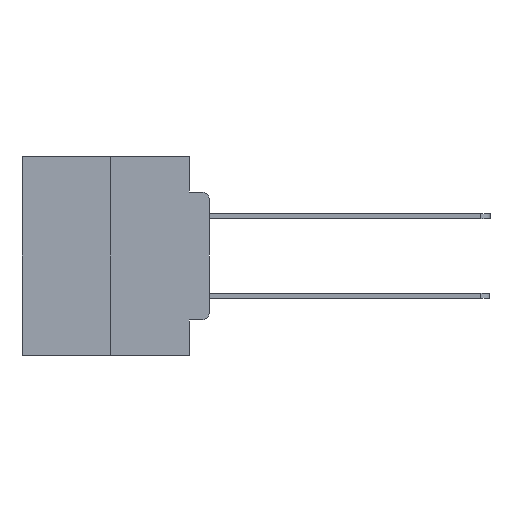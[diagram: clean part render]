
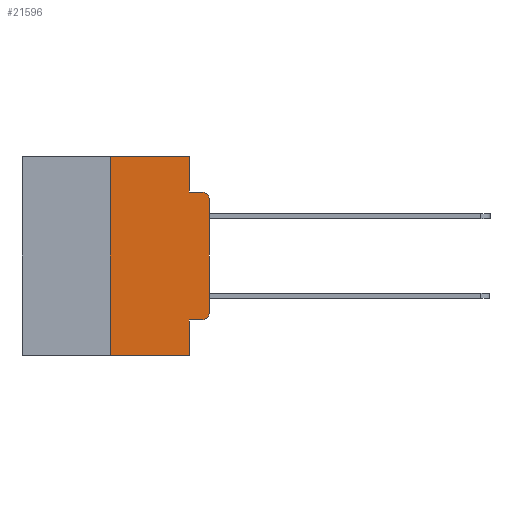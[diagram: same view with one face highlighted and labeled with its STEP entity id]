
A CAD part, left-side view. The second image highlights one B-rep face of the part: STEP entity #21596.
In plain terms, the highlighted planar face has unit normal (-1, 0, 0).
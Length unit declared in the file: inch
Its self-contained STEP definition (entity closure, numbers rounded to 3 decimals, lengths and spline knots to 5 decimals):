
#560 = EDGE_CURVE ( 'NONE', #5393, #11531, #21875, .T. ) ;
#798 = CARTESIAN_POINT ( 'NONE',  ( 0., 0., -0.1085 ) ) ;
#1005 = LINE ( 'NONE', #23950, #6911 ) ;
#1143 = LINE ( 'NONE', #4896, #27524 ) ;
#1494 = ORIENTED_EDGE ( 'NONE', *, *, #15225, .F. ) ;
#2131 = EDGE_CURVE ( 'NONE', #12512, #5947, #9195, .T. ) ;
#2373 = CARTESIAN_POINT ( 'NONE',  ( 0., 0.051, 0. ) ) ;
#2873 = AXIS2_PLACEMENT_3D ( 'NONE', #20112, #7350, #22235 ) ;
#3146 = DIRECTION ( 'NONE',  ( 0., 0., -1. ) ) ;
#3286 = VERTEX_POINT ( 'NONE', #798 ) ;
#3733 = CARTESIAN_POINT ( 'NONE',  ( 0., 0.02, -0.1085 ) ) ;
#3812 = PLANE ( 'NONE',  #27395 ) ;
#4896 = CARTESIAN_POINT ( 'NONE',  ( 0., 0.051, -0.0885 ) ) ;
#4915 = CARTESIAN_POINT ( 'NONE',  ( 0., 0.051, -0.0885 ) ) ;
#4921 = CARTESIAN_POINT ( 'NONE',  ( 0., 0.473, 0. ) ) ;
#4930 = CARTESIAN_POINT ( 'NONE',  ( 0., 0.051, 0. ) ) ;
#5388 = DIRECTION ( 'NONE',  ( 0., 0., 1. ) ) ;
#5393 = VERTEX_POINT ( 'NONE', #4930 ) ;
#5438 = DIRECTION ( 'NONE',  ( 0., 0., 1. ) ) ;
#5648 = DIRECTION ( 'NONE',  ( 0., -1., 0. ) ) ;
#5931 = DIRECTION ( 'NONE',  ( 0., 0., -1. ) ) ;
#5947 = VERTEX_POINT ( 'NONE', #11016 ) ;
#6305 = ORIENTED_EDGE ( 'NONE', *, *, #6551, .F. ) ;
#6402 = CARTESIAN_POINT ( 'NONE',  ( 0., 0.051, -0.4115 ) ) ;
#6551 = EDGE_CURVE ( 'NONE', #12512, #6640, #1005, .T. ) ;
#6640 = VERTEX_POINT ( 'NONE', #11622 ) ;
#6777 = EDGE_CURVE ( 'NONE', #8272, #3286, #12332, .T. ) ;
#6790 = FACE_OUTER_BOUND ( 'NONE', #13102, .T. ) ;
#6911 = VECTOR ( 'NONE', #17625, 39.37008 ) ;
#7350 = DIRECTION ( 'NONE',  ( -1., 0., 0. ) ) ;
#8020 = EDGE_CURVE ( 'NONE', #3286, #26626, #10301, .T. ) ;
#8272 = VERTEX_POINT ( 'NONE', #25757 ) ;
#8650 = DIRECTION ( 'NONE',  ( 0., -1., 0. ) ) ;
#9195 = LINE ( 'NONE', #10422, #19794 ) ;
#9824 = CARTESIAN_POINT ( 'NONE',  ( 0., 0., 0. ) ) ;
#9981 = VERTEX_POINT ( 'NONE', #23063 ) ;
#10078 = ORIENTED_EDGE ( 'NONE', *, *, #25552, .T. ) ;
#10301 = CIRCLE ( 'NONE', #15182, 0.02 ) ;
#10422 = CARTESIAN_POINT ( 'NONE',  ( 0., 0.051, -0.4115 ) ) ;
#10430 = ORIENTED_EDGE ( 'NONE', *, *, #27284, .T. ) ;
#11016 = CARTESIAN_POINT ( 'NONE',  ( 0., 0.02, -0.4115 ) ) ;
#11531 = VERTEX_POINT ( 'NONE', #4915 ) ;
#11622 = CARTESIAN_POINT ( 'NONE',  ( 0., 0.051, -0.5 ) ) ;
#12332 = LINE ( 'NONE', #9824, #22879 ) ;
#12512 = VERTEX_POINT ( 'NONE', #6402 ) ;
#12533 = DIRECTION ( 'NONE',  ( 0., 0., -1. ) ) ;
#13102 = EDGE_LOOP ( 'NONE', ( #17029, #13555, #16099, #14745, #20317, #1494, #10430, #6305, #27192, #10078 ) ) ;
#13258 = CARTESIAN_POINT ( 'NONE',  ( 0., 0.25, -0.5 ) ) ;
#13261 = VERTEX_POINT ( 'NONE', #13258 ) ;
#13336 = EDGE_CURVE ( 'NONE', #9981, #5393, #16441, .T. ) ;
#13555 = ORIENTED_EDGE ( 'NONE', *, *, #8020, .T. ) ;
#13775 = EDGE_CURVE ( 'NONE', #11531, #26626, #1143, .T. ) ;
#13979 = CARTESIAN_POINT ( 'NONE',  ( 0., 0.25, 0. ) ) ;
#14745 = ORIENTED_EDGE ( 'NONE', *, *, #560, .F. ) ;
#15182 = AXIS2_PLACEMENT_3D ( 'NONE', #3733, #18704, #5931 ) ;
#15225 = EDGE_CURVE ( 'NONE', #13261, #9981, #24836, .T. ) ;
#16099 = ORIENTED_EDGE ( 'NONE', *, *, #13775, .F. ) ;
#16441 = LINE ( 'NONE', #4921, #21406 ) ;
#17029 = ORIENTED_EDGE ( 'NONE', *, *, #6777, .T. ) ;
#17625 = DIRECTION ( 'NONE',  ( 0., 0., -1. ) ) ;
#17728 = DIRECTION ( 'NONE',  ( 0., -1., 0. ) ) ;
#18704 = DIRECTION ( 'NONE',  ( -1., 0., 0. ) ) ;
#19106 = CIRCLE ( 'NONE', #2873, 0.02 ) ;
#19290 = VECTOR ( 'NONE', #5388, 39.37008 ) ;
#19794 = VECTOR ( 'NONE', #5648, 39.37008 ) ;
#19862 = DIRECTION ( 'NONE',  ( 0., -1., 0. ) ) ;
#20112 = CARTESIAN_POINT ( 'NONE',  ( 0., 0.02, -0.3915 ) ) ;
#20317 = ORIENTED_EDGE ( 'NONE', *, *, #13336, .F. ) ;
#20928 = CARTESIAN_POINT ( 'NONE',  ( 0., 0.473, 0. ) ) ;
#21210 = CARTESIAN_POINT ( 'NONE',  ( 0., 0.02, -0.0885 ) ) ;
#21356 = CARTESIAN_POINT ( 'NONE',  ( 0., 0.473, -0.5 ) ) ;
#21406 = VECTOR ( 'NONE', #19862, 39.37008 ) ;
#21596 = ADVANCED_FACE ( 'NONE', ( #6790 ), #3812, .F. ) ;
#21875 = LINE ( 'NONE', #2373, #27373 ) ;
#22235 = DIRECTION ( 'NONE',  ( 0., 0., -1. ) ) ;
#22879 = VECTOR ( 'NONE', #5438, 39.37008 ) ;
#23063 = CARTESIAN_POINT ( 'NONE',  ( 0., 0.25, 0. ) ) ;
#23950 = CARTESIAN_POINT ( 'NONE',  ( 0., 0.051, 0. ) ) ;
#24282 = LINE ( 'NONE', #21356, #26888 ) ;
#24836 = LINE ( 'NONE', #13979, #19290 ) ;
#25093 = DIRECTION ( 'NONE',  ( 1., 0., 0. ) ) ;
#25552 = EDGE_CURVE ( 'NONE', #5947, #8272, #19106, .T. ) ;
#25757 = CARTESIAN_POINT ( 'NONE',  ( 0., 0., -0.3915 ) ) ;
#26626 = VERTEX_POINT ( 'NONE', #21210 ) ;
#26888 = VECTOR ( 'NONE', #8650, 39.37008 ) ;
#27192 = ORIENTED_EDGE ( 'NONE', *, *, #2131, .T. ) ;
#27284 = EDGE_CURVE ( 'NONE', #13261, #6640, #24282, .T. ) ;
#27373 = VECTOR ( 'NONE', #3146, 39.37008 ) ;
#27395 = AXIS2_PLACEMENT_3D ( 'NONE', #20928, #25093, #12533 ) ;
#27524 = VECTOR ( 'NONE', #17728, 39.37008 ) ;
